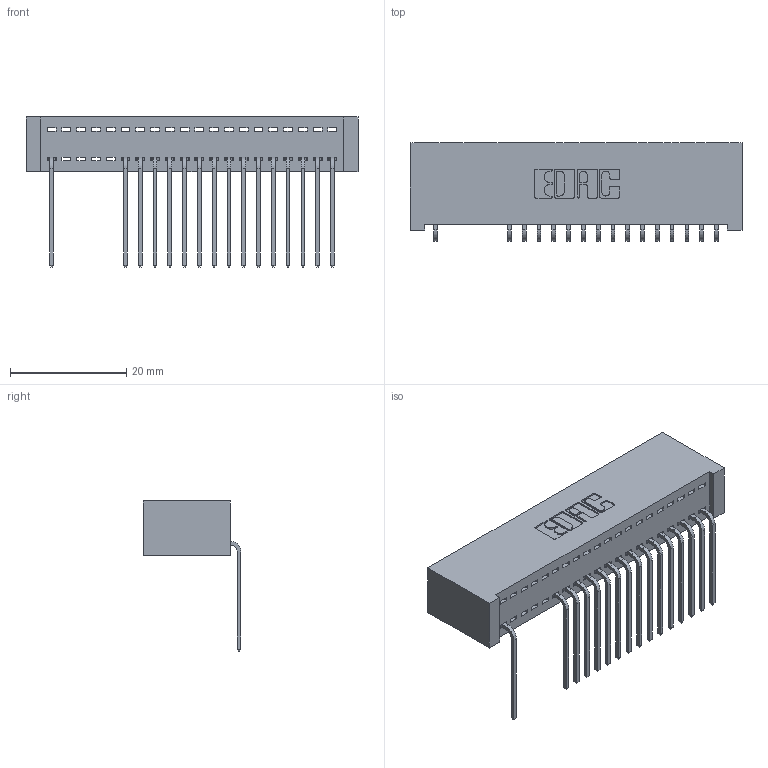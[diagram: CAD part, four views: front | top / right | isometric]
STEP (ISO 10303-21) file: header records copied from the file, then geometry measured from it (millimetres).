
FILE_DESCRIPTION (( 'STEP AP203' ), '1' );
FILE_NAME ('392-020-559-101.STEP', '2018-08-15T07:18:31', ( '' ), ( '' ), 'SwSTEP 2.0', 'SolidWorks 2016', '' );
FILE_SCHEMA (( 'CONFIG_CONTROL_DESIGN' ));
Length unit declared in the file: inch
Products named in the file (3): 392-020-559-101; 342 Part_Lugless; 345-292-001_558 559 Tail - 1
Assembly tree (17 placements, depth 2):
  392-020-559-101
    342 Part_Lugless
    345-292-001_558 559 Tail - 1  x16
Bounding box: 57.05 x 16.83 x 25.78 mm (x, y, z)
Volume: 5337.5 mm3; surface area: 7816.1 mm2
Topology: 17 solids, 17 shells, 1110 faces, 3355 edges, 2214 vertices
Faces by surface type: plane 814, cylinder 296
Entity records: 14619 total; most frequent: CARTESIAN_POINT 2550, ORIENTED_EDGE 2510, DIRECTION 2183, EDGE_CURVE 1255, VECTOR 1135, LINE 1135, VERTEX_POINT 834, AXIS2_PLACEMENT_3D 524
